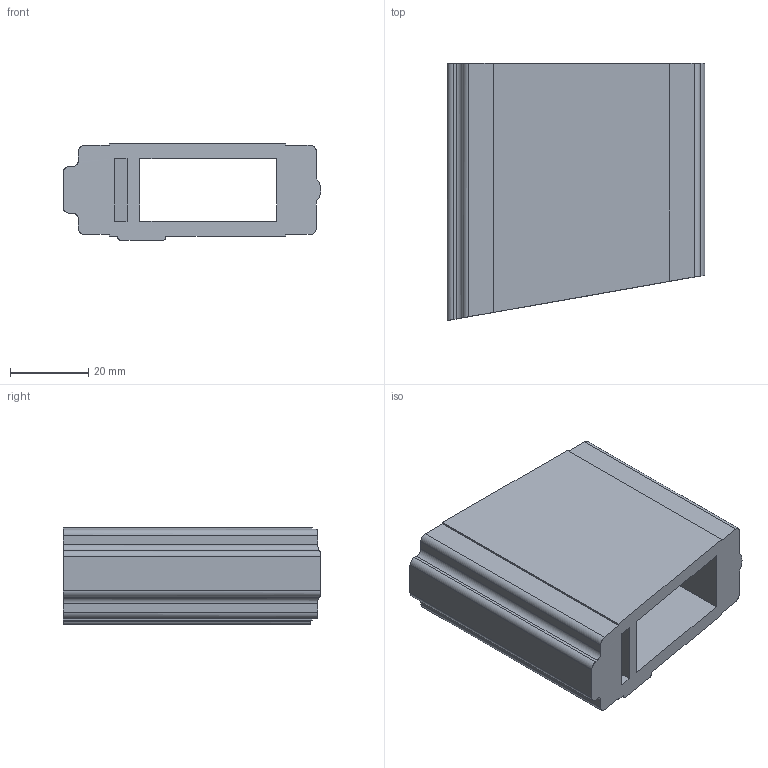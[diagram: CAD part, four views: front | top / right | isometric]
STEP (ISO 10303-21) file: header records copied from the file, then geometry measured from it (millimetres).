
FILE_DESCRIPTION (( 'STEP AP214' ), '1' );
FILE_NAME ('MAG_ADAPTER.STEP', '2013-05-15T15:03:27', ( 'Asher' ), ( '' ), 'SwSTEP 2.0', 'SolidWorks 2013', '' );
FILE_SCHEMA (( 'AUTOMOTIVE_DESIGN' ));
Length unit declared in the file: inch
Products named in the file (1): MAG_ADAPTER
Bounding box: 66.04 x 65.87 x 24.78 mm (x, y, z)
Volume: 55622.1 mm3; surface area: 18835.8 mm2
Topology: 1 solids, 1 shells, 43 faces, 120 edges, 80 vertices
Faces by surface type: plane 32, cylinder 11
Entity records: 1538 total; most frequent: CARTESIAN_POINT 412, ORIENTED_EDGE 240, DIRECTION 204, EDGE_CURVE 120, VECTOR 94, LINE 94, VERTEX_POINT 80, AXIS2_PLACEMENT_3D 55
